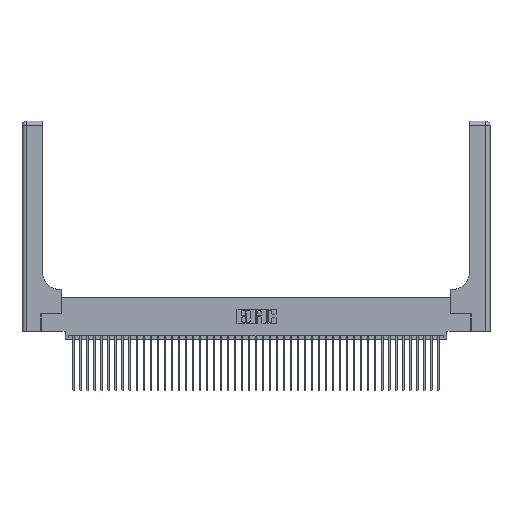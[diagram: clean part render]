
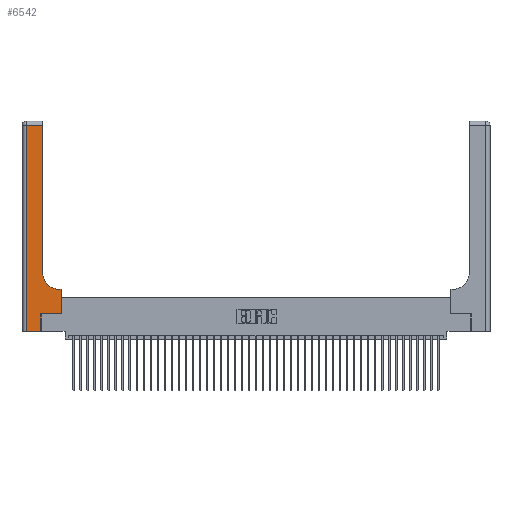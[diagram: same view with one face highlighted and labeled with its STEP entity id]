
A CAD part, top view. The second image highlights one B-rep face of the part: STEP entity #6542.
In plain terms, the highlighted planar face has unit normal (0, 0, 1).
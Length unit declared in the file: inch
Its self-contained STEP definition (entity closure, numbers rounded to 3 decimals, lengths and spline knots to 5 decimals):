
#1282 = LINE ( 'NONE', #36354, #37580 ) ;
#2034 = EDGE_CURVE ( 'NONE', #39485, #5428, #9576, .T. ) ;
#2246 = VECTOR ( 'NONE', #26193, 39.37008 ) ;
#4237 = LINE ( 'NONE', #32025, #40429 ) ;
#4970 = CARTESIAN_POINT ( 'NONE',  ( 0., 0., 0.37 ) ) ;
#5428 = VERTEX_POINT ( 'NONE', #23433 ) ;
#5560 = DIRECTION ( 'NONE',  ( 0., -1., 0. ) ) ;
#5929 = ORIENTED_EDGE ( 'NONE', *, *, #38939, .T. ) ;
#5945 = VERTEX_POINT ( 'NONE', #29451 ) ;
#6440 = EDGE_CURVE ( 'NONE', #24279, #39485, #4237, .T. ) ;
#6542 = ADVANCED_FACE ( 'NONE', ( #21891 ), #28962, .F. ) ;
#7429 = VECTOR ( 'NONE', #5560, 39.37008 ) ;
#7448 = DIRECTION ( 'NONE',  ( 0., 1., 0. ) ) ;
#7973 = VERTEX_POINT ( 'NONE', #25458 ) ;
#9576 = LINE ( 'NONE', #11351, #11751 ) ;
#9724 = CARTESIAN_POINT ( 'NONE',  ( 0.269, 0., 0.37 ) ) ;
#11351 = CARTESIAN_POINT ( 'NONE',  ( 0., 2.94, 0.37 ) ) ;
#11751 = VECTOR ( 'NONE', #35893, 39.37008 ) ;
#12387 = EDGE_CURVE ( 'NONE', #5945, #7973, #20271, .T. ) ;
#12799 = VERTEX_POINT ( 'NONE', #43765 ) ;
#12908 = CARTESIAN_POINT ( 'NONE',  ( 0.5415, 0.6, 0.37 ) ) ;
#12923 = DIRECTION ( 'NONE',  ( 1., 0., 0. ) ) ;
#13240 = DIRECTION ( 'NONE',  ( 0., 1., 0. ) ) ;
#14811 = LINE ( 'NONE', #20382, #41595 ) ;
#16881 = DIRECTION ( 'NONE',  ( -1., 0., 0. ) ) ;
#17525 = ORIENTED_EDGE ( 'NONE', *, *, #36077, .T. ) ;
#18923 = DIRECTION ( 'NONE',  ( 0., 1., 0. ) ) ;
#19792 = CARTESIAN_POINT ( 'NONE',  ( 0.5415, 0.85, 0.37 ) ) ;
#20271 = LINE ( 'NONE', #9724, #43726 ) ;
#20382 = CARTESIAN_POINT ( 'NONE',  ( 0.2915, 0.6, 0.37 ) ) ;
#21891 = FACE_OUTER_BOUND ( 'NONE', #27318, .T. ) ;
#22040 = DIRECTION ( 'NONE',  ( -1., 0., 0. ) ) ;
#22569 = EDGE_CURVE ( 'NONE', #12799, #5945, #39608, .T. ) ;
#23316 = DIRECTION ( 'NONE',  ( 1., 0., 0. ) ) ;
#23433 = CARTESIAN_POINT ( 'NONE',  ( 0.06, 2.94, 0.37 ) ) ;
#24279 = VERTEX_POINT ( 'NONE', #31393 ) ;
#25458 = CARTESIAN_POINT ( 'NONE',  ( 0.269, 0.25, 0.37 ) ) ;
#26193 = DIRECTION ( 'NONE',  ( 1., 0., 0. ) ) ;
#26266 = ORIENTED_EDGE ( 'NONE', *, *, #22569, .T. ) ;
#26640 = CARTESIAN_POINT ( 'NONE',  ( 0.06, 3., 0.37 ) ) ;
#27318 = EDGE_LOOP ( 'NONE', ( #31218, #42600, #43684, #26266, #29573, #5929, #17525, #36131, #29062 ) ) ;
#27956 = VERTEX_POINT ( 'NONE', #12908 ) ;
#28962 = PLANE ( 'NONE',  #35252 ) ;
#29062 = ORIENTED_EDGE ( 'NONE', *, *, #39598, .T. ) ;
#29451 = CARTESIAN_POINT ( 'NONE',  ( 0.269, 0., 0.37 ) ) ;
#29573 = ORIENTED_EDGE ( 'NONE', *, *, #12387, .T. ) ;
#30414 = EDGE_CURVE ( 'NONE', #35827, #27956, #14811, .T. ) ;
#31218 = ORIENTED_EDGE ( 'NONE', *, *, #6440, .T. ) ;
#31393 = CARTESIAN_POINT ( 'NONE',  ( 0.2915, 0.85, 0.37 ) ) ;
#31688 = CARTESIAN_POINT ( 'NONE',  ( 0.5585, 0.6, 0.37 ) ) ;
#32025 = CARTESIAN_POINT ( 'NONE',  ( 0.2915, 3., 0.37 ) ) ;
#33136 = CARTESIAN_POINT ( 'NONE',  ( 0.2915, 2.94, 0.37 ) ) ;
#33964 = CARTESIAN_POINT ( 'NONE',  ( 0.269, 0.25, 0.37 ) ) ;
#34352 = LINE ( 'NONE', #26640, #7429 ) ;
#35252 = AXIS2_PLACEMENT_3D ( 'NONE', #39427, #42924, #22040 ) ;
#35292 = CIRCLE ( 'NONE', #42334, 0.25 ) ;
#35827 = VERTEX_POINT ( 'NONE', #31688 ) ;
#35893 = DIRECTION ( 'NONE',  ( -1., 0., 0. ) ) ;
#36077 = EDGE_CURVE ( 'NONE', #41238, #35827, #1282, .T. ) ;
#36131 = ORIENTED_EDGE ( 'NONE', *, *, #30414, .T. ) ;
#36354 = CARTESIAN_POINT ( 'NONE',  ( 0.5585, 0.25, 0.37 ) ) ;
#37580 = VECTOR ( 'NONE', #18923, 39.37008 ) ;
#38939 = EDGE_CURVE ( 'NONE', #7973, #41238, #42925, .T. ) ;
#39427 = CARTESIAN_POINT ( 'NONE',  ( 0., 3., 0.37 ) ) ;
#39485 = VERTEX_POINT ( 'NONE', #33136 ) ;
#39598 = EDGE_CURVE ( 'NONE', #27956, #24279, #35292, .T. ) ;
#39608 = LINE ( 'NONE', #4970, #2246 ) ;
#40429 = VECTOR ( 'NONE', #7448, 39.37008 ) ;
#41238 = VERTEX_POINT ( 'NONE', #43164 ) ;
#41595 = VECTOR ( 'NONE', #16881, 39.37008 ) ;
#42334 = AXIS2_PLACEMENT_3D ( 'NONE', #19792, #44210, #23316 ) ;
#42600 = ORIENTED_EDGE ( 'NONE', *, *, #2034, .T. ) ;
#42924 = DIRECTION ( 'NONE',  ( 0., 0., -1. ) ) ;
#42925 = LINE ( 'NONE', #33964, #44014 ) ;
#43164 = CARTESIAN_POINT ( 'NONE',  ( 0.5585, 0.25, 0.37 ) ) ;
#43684 = ORIENTED_EDGE ( 'NONE', *, *, #43912, .T. ) ;
#43726 = VECTOR ( 'NONE', #13240, 39.37008 ) ;
#43765 = CARTESIAN_POINT ( 'NONE',  ( 0.06, 0., 0.37 ) ) ;
#43912 = EDGE_CURVE ( 'NONE', #5428, #12799, #34352, .T. ) ;
#44014 = VECTOR ( 'NONE', #12923, 39.37008 ) ;
#44210 = DIRECTION ( 'NONE',  ( 0., 0., -1. ) ) ;
